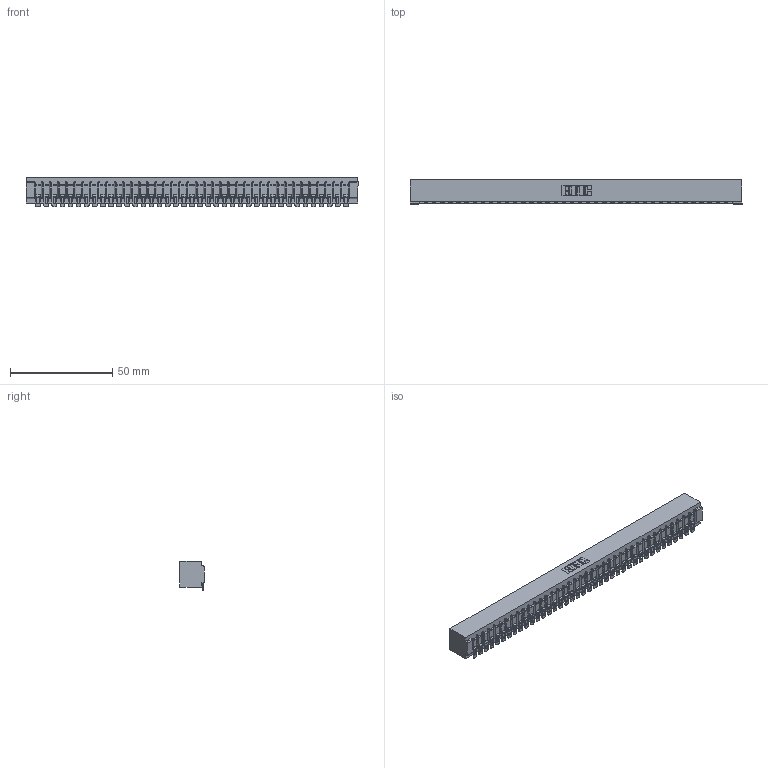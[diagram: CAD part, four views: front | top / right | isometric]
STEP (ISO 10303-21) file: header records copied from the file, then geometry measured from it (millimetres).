
FILE_DESCRIPTION (( 'STEP AP203' ), '1' );
FILE_NAME ('357-039-454-101.STEP', '2020-10-03T04:29:26', ( '' ), ( '' ), 'SwSTEP 2.0', 'SolidWorks 2020', '' );
FILE_SCHEMA (( 'CONFIG_CONTROL_DESIGN' ));
Length unit declared in the file: inch
Products named in the file (3): 357-039-454-101; 307 Part_No Mounting Lugs; 307-290-002_554
Assembly tree (40 placements, depth 2):
  357-039-454-101
    307 Part_No Mounting Lugs
    307-290-002_554  x39
Bounding box: 162.41 x 12.01 x 14.52 mm (x, y, z)
Volume: 17929.1 mm3; surface area: 22977.4 mm2
Topology: 40 solids, 40 shells, 3309 faces, 10166 edges, 6668 vertices
Faces by surface type: plane 1860, cylinder 1369, sphere 80
Entity records: 34491 total; most frequent: CARTESIAN_POINT 5818, ORIENTED_EDGE 5808, DIRECTION 5658, EDGE_CURVE 2904, LINE 2218, VECTOR 2218, VERTEX_POINT 1880, AXIS2_PLACEMENT_3D 1720
